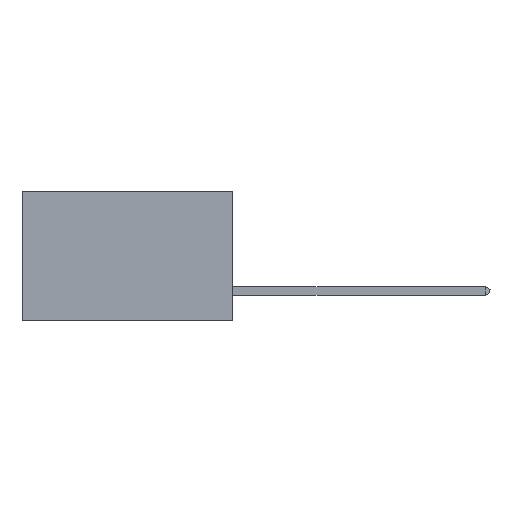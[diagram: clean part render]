
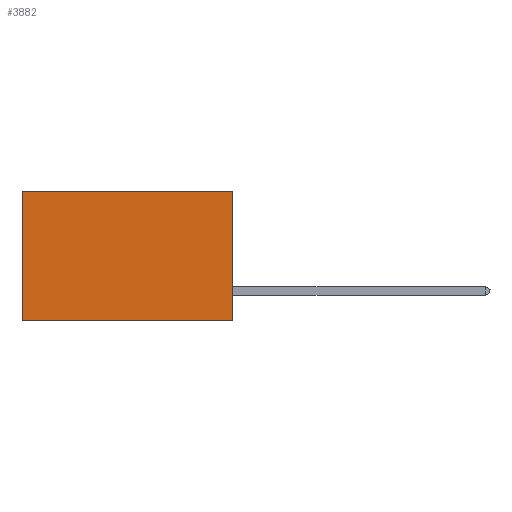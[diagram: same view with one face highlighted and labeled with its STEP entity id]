
A CAD part, left-side view. The second image highlights one B-rep face of the part: STEP entity #3882.
In plain terms, the highlighted planar face has unit normal (-1, 0, 0).
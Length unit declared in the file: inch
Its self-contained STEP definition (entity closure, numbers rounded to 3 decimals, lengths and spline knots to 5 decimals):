
#260 = EDGE_CURVE ( 'NONE', #11223, #31555, #17713, .T. ) ;
#1370 = CARTESIAN_POINT ( 'NONE',  ( 0.2875, 0., -0.37 ) ) ;
#2095 = LINE ( 'NONE', #5882, #34434 ) ;
#2198 = DIRECTION ( 'NONE',  ( 0., 0., -1. ) ) ;
#3882 = ADVANCED_FACE ( 'NONE', ( #14641 ), #26181, .F. ) ;
#5882 = CARTESIAN_POINT ( 'NONE',  ( 0.2875, 0., -0.37 ) ) ;
#6077 = DIRECTION ( 'NONE',  ( 0., 1., 0. ) ) ;
#7531 = DIRECTION ( 'NONE',  ( 0., 0., -1. ) ) ;
#10985 = CARTESIAN_POINT ( 'NONE',  ( 0.2875, 0.6, 0. ) ) ;
#11223 = VERTEX_POINT ( 'NONE', #18516 ) ;
#12821 = VERTEX_POINT ( 'NONE', #28880 ) ;
#13731 = ORIENTED_EDGE ( 'NONE', *, *, #15022, .T. ) ;
#14641 = FACE_OUTER_BOUND ( 'NONE', #16414, .T. ) ;
#15022 = EDGE_CURVE ( 'NONE', #28713, #12821, #34976, .T. ) ;
#16311 = EDGE_CURVE ( 'NONE', #11223, #28713, #18007, .T. ) ;
#16414 = EDGE_LOOP ( 'NONE', ( #13731, #19075, #29324, #18188 ) ) ;
#17713 = LINE ( 'NONE', #32521, #25642 ) ;
#18007 = LINE ( 'NONE', #29687, #34846 ) ;
#18188 = ORIENTED_EDGE ( 'NONE', *, *, #16311, .T. ) ;
#18516 = CARTESIAN_POINT ( 'NONE',  ( 0.2875, 0., 0. ) ) ;
#19075 = ORIENTED_EDGE ( 'NONE', *, *, #28772, .F. ) ;
#20894 = AXIS2_PLACEMENT_3D ( 'NONE', #35590, #26300, #2198 ) ;
#25642 = VECTOR ( 'NONE', #26119, 39.37008 ) ;
#26119 = DIRECTION ( 'NONE',  ( 0., 0., -1. ) ) ;
#26181 = PLANE ( 'NONE',  #20894 ) ;
#26300 = DIRECTION ( 'NONE',  ( 1., 0., 0. ) ) ;
#28713 = VERTEX_POINT ( 'NONE', #10985 ) ;
#28772 = EDGE_CURVE ( 'NONE', #31555, #12821, #2095, .T. ) ;
#28880 = CARTESIAN_POINT ( 'NONE',  ( 0.2875, 0.6, -0.37 ) ) ;
#29324 = ORIENTED_EDGE ( 'NONE', *, *, #260, .F. ) ;
#29687 = CARTESIAN_POINT ( 'NONE',  ( 0.2875, 0., 0. ) ) ;
#31523 = CARTESIAN_POINT ( 'NONE',  ( 0.2875, 0.6, 0. ) ) ;
#31555 = VERTEX_POINT ( 'NONE', #1370 ) ;
#32521 = CARTESIAN_POINT ( 'NONE',  ( 0.2875, 0., 0. ) ) ;
#34434 = VECTOR ( 'NONE', #38462, 39.37008 ) ;
#34846 = VECTOR ( 'NONE', #6077, 39.37008 ) ;
#34976 = LINE ( 'NONE', #31523, #38214 ) ;
#35590 = CARTESIAN_POINT ( 'NONE',  ( 0.2875, 0., 0. ) ) ;
#38214 = VECTOR ( 'NONE', #7531, 39.37008 ) ;
#38462 = DIRECTION ( 'NONE',  ( 0., 1., 0. ) ) ;
